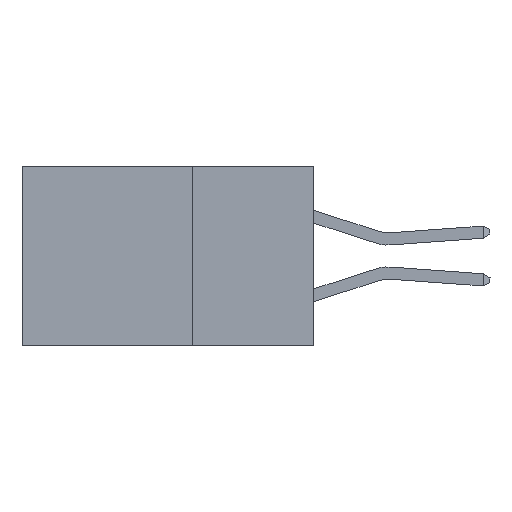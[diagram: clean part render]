
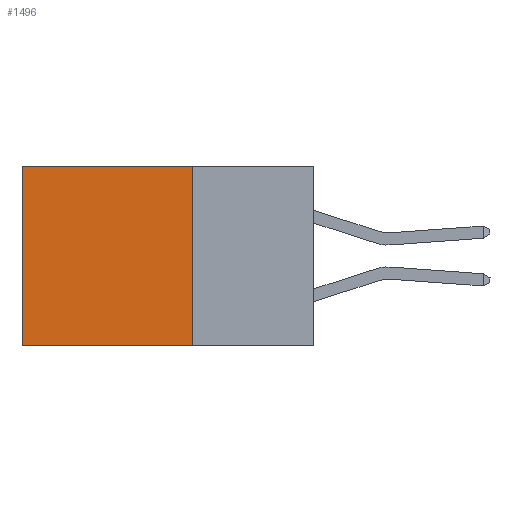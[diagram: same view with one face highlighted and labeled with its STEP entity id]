
A CAD part, left-side view. The second image highlights one B-rep face of the part: STEP entity #1496.
In plain terms, the highlighted planar face has unit normal (-1, 0, 0).
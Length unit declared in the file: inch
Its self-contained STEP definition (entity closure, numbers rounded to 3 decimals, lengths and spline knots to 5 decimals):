
#1496 = ADVANCED_FACE ( 'NONE', ( #21298 ), #7408, .F. ) ;
#2593 = VECTOR ( 'NONE', #14046, 39.37008 ) ;
#2879 = LINE ( 'NONE', #20915, #2593 ) ;
#2963 = VECTOR ( 'NONE', #14217, 39.37008 ) ;
#3460 = LINE ( 'NONE', #19334, #21521 ) ;
#5037 = ORIENTED_EDGE ( 'NONE', *, *, #11960, .F. ) ;
#5063 = DIRECTION ( 'NONE',  ( 0., 1., 0. ) ) ;
#6103 = ORIENTED_EDGE ( 'NONE', *, *, #12283, .T. ) ;
#6936 = VECTOR ( 'NONE', #14220, 39.37008 ) ;
#6996 = CARTESIAN_POINT ( 'NONE',  ( 0.2875, 0.6, 0. ) ) ;
#7356 = ORIENTED_EDGE ( 'NONE', *, *, #13537, .T. ) ;
#7408 = PLANE ( 'NONE',  #8858 ) ;
#7859 = VERTEX_POINT ( 'NONE', #9872 ) ;
#7868 = DIRECTION ( 'NONE',  ( 0., 0., -1. ) ) ;
#8743 = CARTESIAN_POINT ( 'NONE',  ( 0.2875, 0.25, -0.37 ) ) ;
#8818 = VERTEX_POINT ( 'NONE', #8743 ) ;
#8858 = AXIS2_PLACEMENT_3D ( 'NONE', #12900, #20015, #7868 ) ;
#9872 = CARTESIAN_POINT ( 'NONE',  ( 0.2875, 0.6, -0.37 ) ) ;
#9902 = EDGE_CURVE ( 'NONE', #10822, #8818, #13660, .T. ) ;
#10822 = VERTEX_POINT ( 'NONE', #15500 ) ;
#11960 = EDGE_CURVE ( 'NONE', #8818, #7859, #3460, .T. ) ;
#12283 = EDGE_CURVE ( 'NONE', #10822, #13878, #2879, .T. ) ;
#12900 = CARTESIAN_POINT ( 'NONE',  ( 0.2875, 0.25, 0. ) ) ;
#13240 = LINE ( 'NONE', #15827, #6936 ) ;
#13406 = ORIENTED_EDGE ( 'NONE', *, *, #9902, .F. ) ;
#13537 = EDGE_CURVE ( 'NONE', #13878, #7859, #13240, .T. ) ;
#13660 = LINE ( 'NONE', #15907, #2963 ) ;
#13878 = VERTEX_POINT ( 'NONE', #6996 ) ;
#14046 = DIRECTION ( 'NONE',  ( 0., 1., 0. ) ) ;
#14217 = DIRECTION ( 'NONE',  ( 0., 0., -1. ) ) ;
#14220 = DIRECTION ( 'NONE',  ( 0., 0., -1. ) ) ;
#15082 = EDGE_LOOP ( 'NONE', ( #7356, #5037, #13406, #6103 ) ) ;
#15500 = CARTESIAN_POINT ( 'NONE',  ( 0.2875, 0.25, 0. ) ) ;
#15827 = CARTESIAN_POINT ( 'NONE',  ( 0.2875, 0.6, 0. ) ) ;
#15907 = CARTESIAN_POINT ( 'NONE',  ( 0.2875, 0.25, 0. ) ) ;
#19334 = CARTESIAN_POINT ( 'NONE',  ( 0.2875, 0.25, -0.37 ) ) ;
#20015 = DIRECTION ( 'NONE',  ( 1., 0., 0. ) ) ;
#20915 = CARTESIAN_POINT ( 'NONE',  ( 0.2875, 0.25, 0. ) ) ;
#21298 = FACE_OUTER_BOUND ( 'NONE', #15082, .T. ) ;
#21521 = VECTOR ( 'NONE', #5063, 39.37008 ) ;
